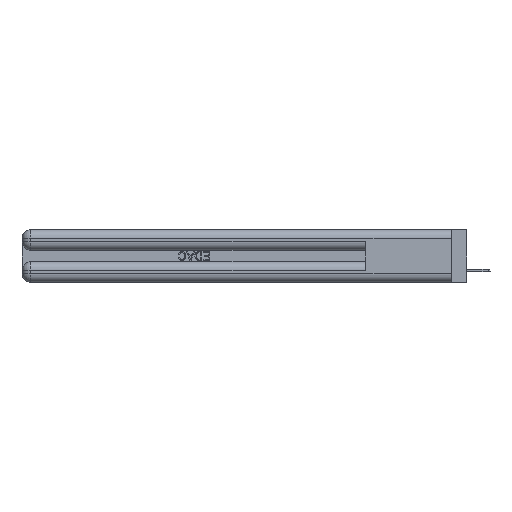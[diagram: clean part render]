
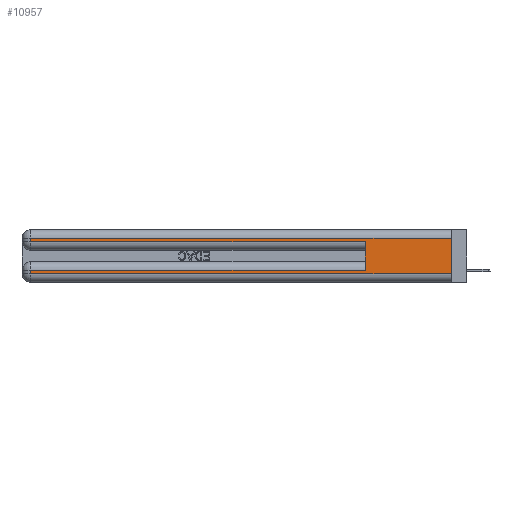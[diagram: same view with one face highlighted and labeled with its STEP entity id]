
A CAD part, left-side view. The second image highlights one B-rep face of the part: STEP entity #10957.
In plain terms, the highlighted planar face has unit normal (-1, 0, 0).
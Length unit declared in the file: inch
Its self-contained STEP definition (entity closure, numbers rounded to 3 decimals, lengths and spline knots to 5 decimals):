
#61 = VERTEX_POINT ( 'NONE', #22259 ) ;
#1775 = VECTOR ( 'NONE', #42029, 39.37008 ) ;
#2209 = EDGE_CURVE ( 'NONE', #44656, #23422, #24818, .T. ) ;
#2380 = VERTEX_POINT ( 'NONE', #40986 ) ;
#2722 = CARTESIAN_POINT ( 'NONE',  ( 0., 2.94, 0.085 ) ) ;
#4012 = EDGE_CURVE ( 'NONE', #44656, #2380, #46592, .T. ) ;
#4238 = VECTOR ( 'NONE', #43350, 39.37008 ) ;
#4619 = EDGE_CURVE ( 'NONE', #16415, #39017, #45332, .T. ) ;
#4938 = CARTESIAN_POINT ( 'NONE',  ( 0., 0., 0.31 ) ) ;
#5078 = VECTOR ( 'NONE', #30837, 39.37008 ) ;
#5403 = DIRECTION ( 'NONE',  ( 0., 0., -1. ) ) ;
#6290 = LINE ( 'NONE', #20202, #5078 ) ;
#6729 = EDGE_CURVE ( 'NONE', #23422, #32042, #42298, .T. ) ;
#8330 = CARTESIAN_POINT ( 'NONE',  ( 0., 0., 0.37 ) ) ;
#10957 = ADVANCED_FACE ( 'NONE', ( #40054 ), #16191, .F. ) ;
#11833 = ORIENTED_EDGE ( 'NONE', *, *, #17874, .T. ) ;
#12149 = CARTESIAN_POINT ( 'NONE',  ( 0., 0., 0.285 ) ) ;
#13009 = ORIENTED_EDGE ( 'NONE', *, *, #4619, .T. ) ;
#13472 = LINE ( 'NONE', #35957, #4238 ) ;
#14871 = ORIENTED_EDGE ( 'NONE', *, *, #2209, .T. ) ;
#15307 = CARTESIAN_POINT ( 'NONE',  ( 0., 0., 0.31 ) ) ;
#15673 = DIRECTION ( 'NONE',  ( 1., 0., 0. ) ) ;
#16191 = PLANE ( 'NONE',  #17041 ) ;
#16415 = VERTEX_POINT ( 'NONE', #2722 ) ;
#16444 = ORIENTED_EDGE ( 'NONE', *, *, #6729, .T. ) ;
#17041 = AXIS2_PLACEMENT_3D ( 'NONE', #8330, #15673, #45596 ) ;
#17225 = VECTOR ( 'NONE', #23750, 39.37008 ) ;
#17874 = EDGE_CURVE ( 'NONE', #32042, #43927, #18054, .T. ) ;
#18054 = LINE ( 'NONE', #12149, #21519 ) ;
#19242 = VECTOR ( 'NONE', #5403, 39.37008 ) ;
#19764 = CARTESIAN_POINT ( 'NONE',  ( 0., 0.6, 0.145 ) ) ;
#20202 = CARTESIAN_POINT ( 'NONE',  ( 0., 0., 0.06 ) ) ;
#21046 = DIRECTION ( 'NONE',  ( 0., 0., 1. ) ) ;
#21519 = VECTOR ( 'NONE', #34463, 39.37008 ) ;
#22259 = CARTESIAN_POINT ( 'NONE',  ( 0., 0.6, 0.085 ) ) ;
#22811 = EDGE_CURVE ( 'NONE', #61, #43927, #32414, .T. ) ;
#23408 = EDGE_CURVE ( 'NONE', #39017, #2380, #6290, .T. ) ;
#23422 = VERTEX_POINT ( 'NONE', #23917 ) ;
#23750 = DIRECTION ( 'NONE',  ( 0., 0., -1. ) ) ;
#23917 = CARTESIAN_POINT ( 'NONE',  ( 0., 2.94, 0.31 ) ) ;
#24064 = CARTESIAN_POINT ( 'NONE',  ( 0., 0., 0.37 ) ) ;
#24818 = LINE ( 'NONE', #4938, #1775 ) ;
#26798 = ORIENTED_EDGE ( 'NONE', *, *, #4012, .F. ) ;
#26946 = CARTESIAN_POINT ( 'NONE',  ( 0., 2.94, 0.37 ) ) ;
#30084 = EDGE_CURVE ( 'NONE', #61, #16415, #13472, .T. ) ;
#30837 = DIRECTION ( 'NONE',  ( 0., -1., 0. ) ) ;
#31696 = ORIENTED_EDGE ( 'NONE', *, *, #23408, .T. ) ;
#31848 = VECTOR ( 'NONE', #21046, 39.37008 ) ;
#32042 = VERTEX_POINT ( 'NONE', #43831 ) ;
#32178 = ORIENTED_EDGE ( 'NONE', *, *, #22811, .F. ) ;
#32414 = LINE ( 'NONE', #19764, #31848 ) ;
#34463 = DIRECTION ( 'NONE',  ( 0., -1., 0. ) ) ;
#35957 = CARTESIAN_POINT ( 'NONE',  ( 0., 0., 0.085 ) ) ;
#39017 = VERTEX_POINT ( 'NONE', #46595 ) ;
#39134 = VECTOR ( 'NONE', #45703, 39.37008 ) ;
#39491 = EDGE_LOOP ( 'NONE', ( #26798, #14871, #16444, #11833, #32178, #45317, #13009, #31696 ) ) ;
#40054 = FACE_OUTER_BOUND ( 'NONE', #39491, .T. ) ;
#40986 = CARTESIAN_POINT ( 'NONE',  ( 0., 0., 0.06 ) ) ;
#42029 = DIRECTION ( 'NONE',  ( 0., 1., 0. ) ) ;
#42298 = LINE ( 'NONE', #46185, #19242 ) ;
#43350 = DIRECTION ( 'NONE',  ( 0., 1., 0. ) ) ;
#43831 = CARTESIAN_POINT ( 'NONE',  ( 0., 2.94, 0.285 ) ) ;
#43927 = VERTEX_POINT ( 'NONE', #44124 ) ;
#44124 = CARTESIAN_POINT ( 'NONE',  ( 0., 0.6, 0.285 ) ) ;
#44656 = VERTEX_POINT ( 'NONE', #15307 ) ;
#45317 = ORIENTED_EDGE ( 'NONE', *, *, #30084, .T. ) ;
#45332 = LINE ( 'NONE', #26946, #17225 ) ;
#45596 = DIRECTION ( 'NONE',  ( 0., 0., -1. ) ) ;
#45703 = DIRECTION ( 'NONE',  ( 0., 0., -1. ) ) ;
#46185 = CARTESIAN_POINT ( 'NONE',  ( 0., 2.94, 0.37 ) ) ;
#46592 = LINE ( 'NONE', #24064, #39134 ) ;
#46595 = CARTESIAN_POINT ( 'NONE',  ( 0., 2.94, 0.06 ) ) ;
